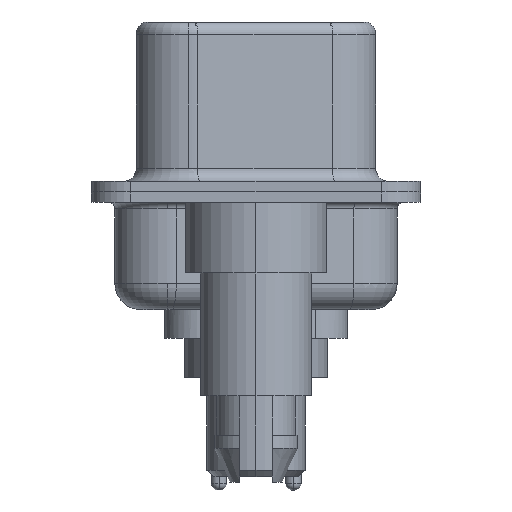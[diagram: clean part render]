
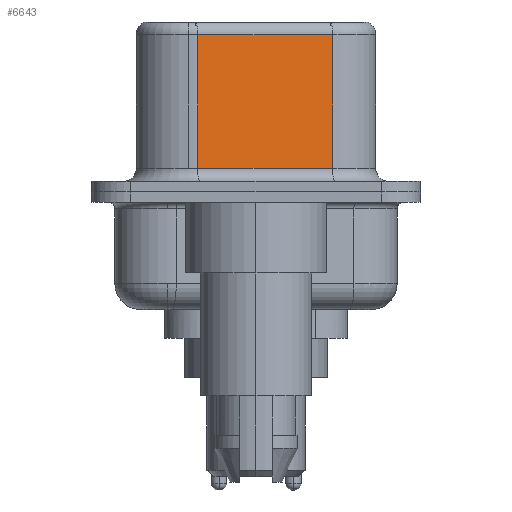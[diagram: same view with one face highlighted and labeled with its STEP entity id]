
A CAD part, left-side view. The second image highlights one B-rep face of the part: STEP entity #6643.
In plain terms, the highlighted planar face has unit normal (-0.985, -0.174, 0).
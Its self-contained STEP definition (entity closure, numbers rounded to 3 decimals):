
#671 = DIRECTION ( 'NONE',  ( -0.174, 0.985, 0. ) ) ;
#871 = EDGE_CURVE ( 'NONE', #17037, #10068, #1713, .T. ) ;
#1366 = LINE ( 'NONE', #18238, #20153 ) ;
#1713 = LINE ( 'NONE', #13944, #19320 ) ;
#5296 = VECTOR ( 'NONE', #671, 1000. ) ;
#6184 = AXIS2_PLACEMENT_3D ( 'NONE', #18859, #13457, #11931 ) ;
#6643 = ADVANCED_FACE ( 'NONE', ( #10985 ), #13543, .F. ) ;
#7151 = VECTOR ( 'NONE', #19149, 1000. ) ;
#7328 = DIRECTION ( 'NONE',  ( 0.174, -0.985, 0. ) ) ;
#7709 = DIRECTION ( 'NONE',  ( 0., 0., -1. ) ) ;
#8081 = CARTESIAN_POINT ( 'NONE',  ( 4.58, -2.927, 6.52 ) ) ;
#8493 = ORIENTED_EDGE ( 'NONE', *, *, #14469, .T. ) ;
#9213 = EDGE_CURVE ( 'NONE', #9781, #19135, #12002, .T. ) ;
#9214 = EDGE_LOOP ( 'NONE', ( #22679, #8493, #14691, #10226 ) ) ;
#9781 = VERTEX_POINT ( 'NONE', #15225 ) ;
#10065 = CARTESIAN_POINT ( 'NONE',  ( 4.58, -2.927, 0.9 ) ) ;
#10068 = VERTEX_POINT ( 'NONE', #19753 ) ;
#10131 = LINE ( 'NONE', #18756, #5296 ) ;
#10226 = ORIENTED_EDGE ( 'NONE', *, *, #23370, .T. ) ;
#10985 = FACE_OUTER_BOUND ( 'NONE', #9214, .T. ) ;
#11931 = DIRECTION ( 'NONE',  ( -0.174, 0.985, 0. ) ) ;
#12002 = LINE ( 'NONE', #8081, #7151 ) ;
#13457 = DIRECTION ( 'NONE',  ( 0.985, 0.174, 0. ) ) ;
#13543 = PLANE ( 'NONE',  #6184 ) ;
#13944 = CARTESIAN_POINT ( 'NONE',  ( 3.67, 2.233, 6.52 ) ) ;
#14469 = EDGE_CURVE ( 'NONE', #9781, #17037, #10131, .T. ) ;
#14691 = ORIENTED_EDGE ( 'NONE', *, *, #871, .T. ) ;
#15225 = CARTESIAN_POINT ( 'NONE',  ( 4.58, -2.927, 6.02 ) ) ;
#17037 = VERTEX_POINT ( 'NONE', #22221 ) ;
#18238 = CARTESIAN_POINT ( 'NONE',  ( 4.58, -2.927, 0.9 ) ) ;
#18756 = CARTESIAN_POINT ( 'NONE',  ( 4.58, -2.927, 6.02 ) ) ;
#18859 = CARTESIAN_POINT ( 'NONE',  ( 4.58, -2.927, 6.52 ) ) ;
#19135 = VERTEX_POINT ( 'NONE', #10065 ) ;
#19149 = DIRECTION ( 'NONE',  ( 0., 0., -1. ) ) ;
#19320 = VECTOR ( 'NONE', #7709, 1000. ) ;
#19753 = CARTESIAN_POINT ( 'NONE',  ( 3.67, 2.233, 0.9 ) ) ;
#20153 = VECTOR ( 'NONE', #7328, 1000. ) ;
#22221 = CARTESIAN_POINT ( 'NONE',  ( 3.67, 2.233, 6.02 ) ) ;
#22679 = ORIENTED_EDGE ( 'NONE', *, *, #9213, .F. ) ;
#23370 = EDGE_CURVE ( 'NONE', #10068, #19135, #1366, .T. ) ;
